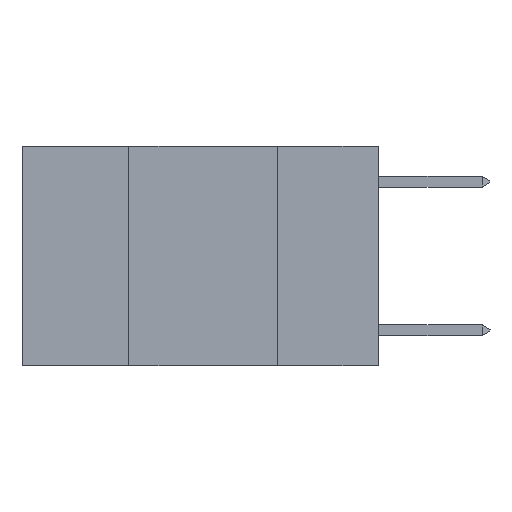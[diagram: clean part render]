
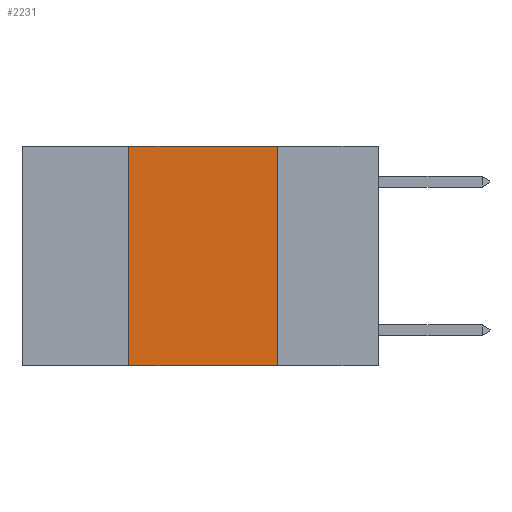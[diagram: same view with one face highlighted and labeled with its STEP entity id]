
A CAD part, left-side view. The second image highlights one B-rep face of the part: STEP entity #2231.
In plain terms, the highlighted planar face has unit normal (-1, 0, 0).
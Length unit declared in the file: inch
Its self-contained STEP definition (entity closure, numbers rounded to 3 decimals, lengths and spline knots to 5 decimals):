
#2231 = ADVANCED_FACE ( 'NONE', ( #23274 ), #11334, .F. ) ;
#2544 = CARTESIAN_POINT ( 'NONE',  ( 0., 0.6, -0.37 ) ) ;
#4038 = VERTEX_POINT ( 'NONE', #21414 ) ;
#4757 = EDGE_LOOP ( 'NONE', ( #13451, #13768, #14228, #14252 ) ) ;
#4993 = DIRECTION ( 'NONE',  ( 0., -1., 0. ) ) ;
#7748 = EDGE_CURVE ( 'NONE', #19412, #10271, #23813, .T. ) ;
#8080 = VERTEX_POINT ( 'NONE', #21167 ) ;
#9901 = LINE ( 'NONE', #11325, #25413 ) ;
#10271 = VERTEX_POINT ( 'NONE', #16902 ) ;
#11244 = DIRECTION ( 'NONE',  ( 0., 0., -1. ) ) ;
#11265 = DIRECTION ( 'NONE',  ( 1., 0., 0. ) ) ;
#11325 = CARTESIAN_POINT ( 'NONE',  ( 0., 0.42, 0. ) ) ;
#11330 = CARTESIAN_POINT ( 'NONE',  ( 0., 0.6, 0. ) ) ;
#11334 = PLANE ( 'NONE',  #19413 ) ;
#12312 = EDGE_CURVE ( 'NONE', #8080, #19412, #23931, .T. ) ;
#13451 = ORIENTED_EDGE ( 'NONE', *, *, #7748, .F. ) ;
#13768 = ORIENTED_EDGE ( 'NONE', *, *, #12312, .F. ) ;
#14228 = ORIENTED_EDGE ( 'NONE', *, *, #25278, .F. ) ;
#14252 = ORIENTED_EDGE ( 'NONE', *, *, #22513, .T. ) ;
#15626 = DIRECTION ( 'NONE',  ( 0., 0., 1. ) ) ;
#16746 = LINE ( 'NONE', #2544, #27680 ) ;
#16902 = CARTESIAN_POINT ( 'NONE',  ( 0., 0.17, -0.37 ) ) ;
#17985 = CARTESIAN_POINT ( 'NONE',  ( 0., 0.17, 0. ) ) ;
#19412 = VERTEX_POINT ( 'NONE', #17985 ) ;
#19413 = AXIS2_PLACEMENT_3D ( 'NONE', #11330, #11265, #11244 ) ;
#19888 = DIRECTION ( 'NONE',  ( 0., -1., 0. ) ) ;
#20043 = CARTESIAN_POINT ( 'NONE',  ( 0., 0.6, 0. ) ) ;
#21167 = CARTESIAN_POINT ( 'NONE',  ( 0., 0.42, 0. ) ) ;
#21414 = CARTESIAN_POINT ( 'NONE',  ( 0., 0.42, -0.37 ) ) ;
#22513 = EDGE_CURVE ( 'NONE', #4038, #10271, #16746, .T. ) ;
#23274 = FACE_OUTER_BOUND ( 'NONE', #4757, .T. ) ;
#23789 = VECTOR ( 'NONE', #25114, 39.37008 ) ;
#23813 = LINE ( 'NONE', #25091, #23789 ) ;
#23885 = VECTOR ( 'NONE', #4993, 39.37008 ) ;
#23931 = LINE ( 'NONE', #20043, #23885 ) ;
#25091 = CARTESIAN_POINT ( 'NONE',  ( 0., 0.17, 0. ) ) ;
#25114 = DIRECTION ( 'NONE',  ( 0., 0., -1. ) ) ;
#25278 = EDGE_CURVE ( 'NONE', #4038, #8080, #9901, .T. ) ;
#25413 = VECTOR ( 'NONE', #15626, 39.37008 ) ;
#27680 = VECTOR ( 'NONE', #19888, 39.37008 ) ;
